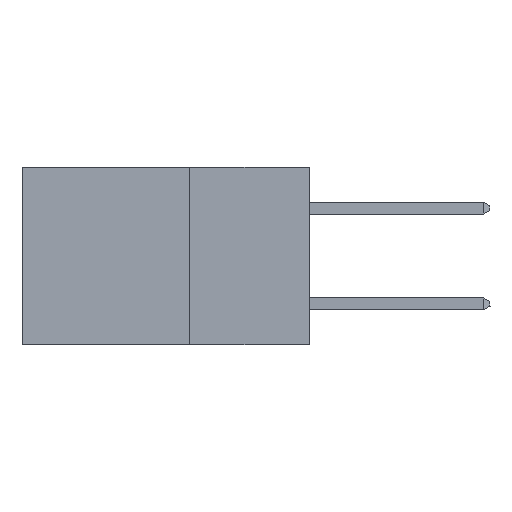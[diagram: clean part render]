
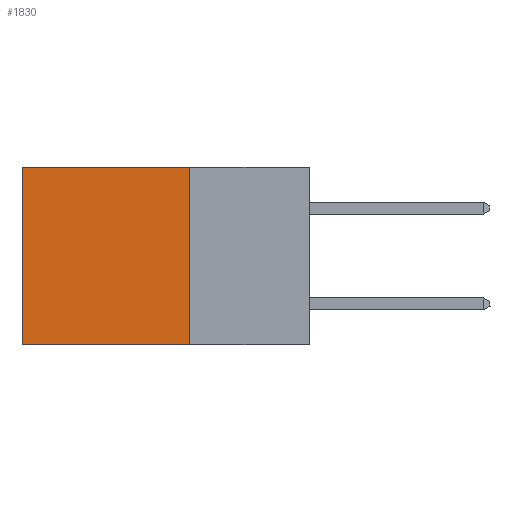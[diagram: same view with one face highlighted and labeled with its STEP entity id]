
A CAD part, left-side view. The second image highlights one B-rep face of the part: STEP entity #1830.
In plain terms, the highlighted planar face has unit normal (-1, 0, 0).
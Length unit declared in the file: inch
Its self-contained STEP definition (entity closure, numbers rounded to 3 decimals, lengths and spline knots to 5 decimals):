
#235 = CARTESIAN_POINT ( 'NONE',  ( 0.2875, 0.6, 0. ) ) ;
#253 = VERTEX_POINT ( 'NONE', #10298 ) ;
#579 = VERTEX_POINT ( 'NONE', #235 ) ;
#1241 = AXIS2_PLACEMENT_3D ( 'NONE', #5737, #5658, #5641 ) ;
#1697 = VERTEX_POINT ( 'NONE', #7047 ) ;
#1830 = ADVANCED_FACE ( 'NONE', ( #2599 ), #5877, .F. ) ;
#2197 = LINE ( 'NONE', #2470, #10637 ) ;
#2425 = DIRECTION ( 'NONE',  ( 0., 0., -1. ) ) ;
#2470 = CARTESIAN_POINT ( 'NONE',  ( 0.2875, 0.6, 0. ) ) ;
#2599 = FACE_OUTER_BOUND ( 'NONE', #5387, .T. ) ;
#3041 = CARTESIAN_POINT ( 'NONE',  ( 0.2875, 0.25, 0. ) ) ;
#3097 = DIRECTION ( 'NONE',  ( 0., 1., 0. ) ) ;
#3320 = EDGE_CURVE ( 'NONE', #253, #1697, #10301, .T. ) ;
#3724 = EDGE_CURVE ( 'NONE', #579, #1697, #2197, .T. ) ;
#4469 = ORIENTED_EDGE ( 'NONE', *, *, #3724, .T. ) ;
#5387 = EDGE_LOOP ( 'NONE', ( #4469, #11322, #11686, #12343 ) ) ;
#5641 = DIRECTION ( 'NONE',  ( 0., 0., -1. ) ) ;
#5658 = DIRECTION ( 'NONE',  ( 1., 0., 0. ) ) ;
#5737 = CARTESIAN_POINT ( 'NONE',  ( 0.2875, 0.25, 0. ) ) ;
#5877 = PLANE ( 'NONE',  #1241 ) ;
#7011 = CARTESIAN_POINT ( 'NONE',  ( 0.2875, 0.25, -0.37 ) ) ;
#7047 = CARTESIAN_POINT ( 'NONE',  ( 0.2875, 0.6, -0.37 ) ) ;
#7068 = EDGE_CURVE ( 'NONE', #11951, #253, #13588, .T. ) ;
#7089 = DIRECTION ( 'NONE',  ( 0., 1., 0. ) ) ;
#7816 = VECTOR ( 'NONE', #9586, 39.37008 ) ;
#8398 = EDGE_CURVE ( 'NONE', #11951, #579, #10748, .T. ) ;
#8429 = CARTESIAN_POINT ( 'NONE',  ( 0.2875, 0.25, 0. ) ) ;
#9586 = DIRECTION ( 'NONE',  ( 0., 0., -1. ) ) ;
#9976 = VECTOR ( 'NONE', #7089, 39.37008 ) ;
#10298 = CARTESIAN_POINT ( 'NONE',  ( 0.2875, 0.25, -0.37 ) ) ;
#10301 = LINE ( 'NONE', #7011, #9976 ) ;
#10637 = VECTOR ( 'NONE', #2425, 39.37008 ) ;
#10748 = LINE ( 'NONE', #10768, #11069 ) ;
#10768 = CARTESIAN_POINT ( 'NONE',  ( 0.2875, 0.25, 0. ) ) ;
#11069 = VECTOR ( 'NONE', #3097, 39.37008 ) ;
#11322 = ORIENTED_EDGE ( 'NONE', *, *, #3320, .F. ) ;
#11686 = ORIENTED_EDGE ( 'NONE', *, *, #7068, .F. ) ;
#11951 = VERTEX_POINT ( 'NONE', #3041 ) ;
#12343 = ORIENTED_EDGE ( 'NONE', *, *, #8398, .T. ) ;
#13588 = LINE ( 'NONE', #8429, #7816 ) ;
